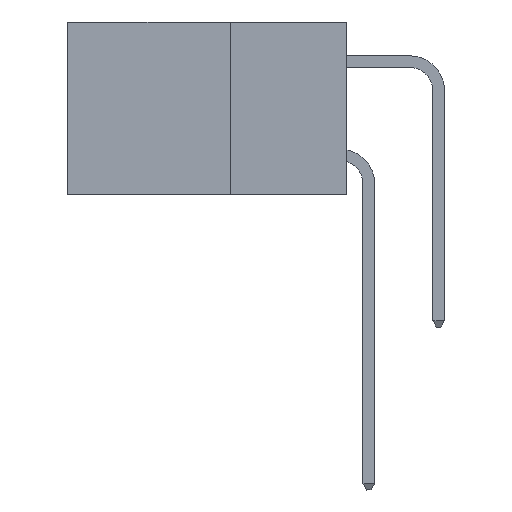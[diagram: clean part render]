
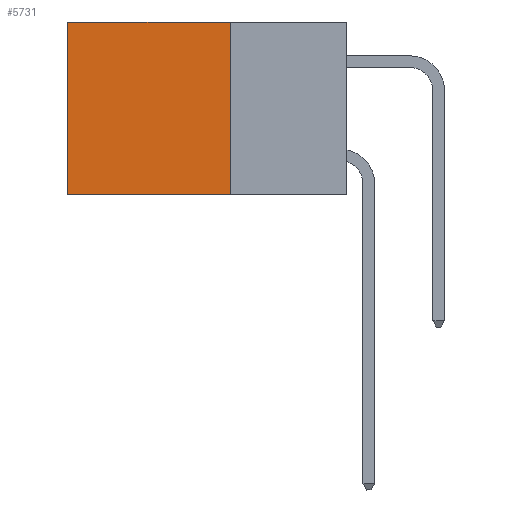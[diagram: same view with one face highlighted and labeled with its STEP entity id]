
A CAD part, left-side view. The second image highlights one B-rep face of the part: STEP entity #5731.
In plain terms, the highlighted planar face has unit normal (-1, 0, 0).
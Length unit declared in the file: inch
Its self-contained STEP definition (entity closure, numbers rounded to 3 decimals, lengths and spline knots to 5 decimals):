
#300 = DIRECTION ( 'NONE',  ( 0., 1., 0. ) ) ;
#339 = EDGE_CURVE ( 'NONE', #11850, #1964, #5394, .T. ) ;
#1342 = DIRECTION ( 'NONE',  ( 0., 1., 0. ) ) ;
#1818 = VERTEX_POINT ( 'NONE', #2276 ) ;
#1964 = VERTEX_POINT ( 'NONE', #11108 ) ;
#2276 = CARTESIAN_POINT ( 'NONE',  ( 0.2875, 0.25, 0. ) ) ;
#2569 = VECTOR ( 'NONE', #2847, 39.37008 ) ;
#2829 = VECTOR ( 'NONE', #1342, 39.37008 ) ;
#2847 = DIRECTION ( 'NONE',  ( 0., 0., -1. ) ) ;
#2976 = EDGE_CURVE ( 'NONE', #8353, #1964, #3610, .T. ) ;
#3076 = EDGE_LOOP ( 'NONE', ( #4295, #9761, #5163, #5440 ) ) ;
#3610 = LINE ( 'NONE', #11179, #2829 ) ;
#4295 = ORIENTED_EDGE ( 'NONE', *, *, #339, .T. ) ;
#4810 = DIRECTION ( 'NONE',  ( 1., 0., 0. ) ) ;
#5008 = PLANE ( 'NONE',  #5174 ) ;
#5163 = ORIENTED_EDGE ( 'NONE', *, *, #11243, .F. ) ;
#5174 = AXIS2_PLACEMENT_3D ( 'NONE', #10856, #4810, #13323 ) ;
#5375 = VECTOR ( 'NONE', #300, 39.37008 ) ;
#5394 = LINE ( 'NONE', #12882, #14369 ) ;
#5440 = ORIENTED_EDGE ( 'NONE', *, *, #12993, .T. ) ;
#5731 = ADVANCED_FACE ( 'NONE', ( #9426 ), #5008, .F. ) ;
#7538 = CARTESIAN_POINT ( 'NONE',  ( 0.2875, 0.25, 0. ) ) ;
#8230 = LINE ( 'NONE', #13559, #5375 ) ;
#8353 = VERTEX_POINT ( 'NONE', #11332 ) ;
#9426 = FACE_OUTER_BOUND ( 'NONE', #3076, .T. ) ;
#9509 = DIRECTION ( 'NONE',  ( 0., 0., -1. ) ) ;
#9761 = ORIENTED_EDGE ( 'NONE', *, *, #2976, .F. ) ;
#10856 = CARTESIAN_POINT ( 'NONE',  ( 0.2875, 0.25, 0. ) ) ;
#11108 = CARTESIAN_POINT ( 'NONE',  ( 0.2875, 0.6, -0.37 ) ) ;
#11179 = CARTESIAN_POINT ( 'NONE',  ( 0.2875, 0.25, -0.37 ) ) ;
#11243 = EDGE_CURVE ( 'NONE', #1818, #8353, #11328, .T. ) ;
#11328 = LINE ( 'NONE', #7538, #2569 ) ;
#11332 = CARTESIAN_POINT ( 'NONE',  ( 0.2875, 0.25, -0.37 ) ) ;
#11850 = VERTEX_POINT ( 'NONE', #11990 ) ;
#11990 = CARTESIAN_POINT ( 'NONE',  ( 0.2875, 0.6, 0. ) ) ;
#12882 = CARTESIAN_POINT ( 'NONE',  ( 0.2875, 0.6, 0. ) ) ;
#12993 = EDGE_CURVE ( 'NONE', #1818, #11850, #8230, .T. ) ;
#13323 = DIRECTION ( 'NONE',  ( 0., 0., -1. ) ) ;
#13559 = CARTESIAN_POINT ( 'NONE',  ( 0.2875, 0.25, 0. ) ) ;
#14369 = VECTOR ( 'NONE', #9509, 39.37008 ) ;
